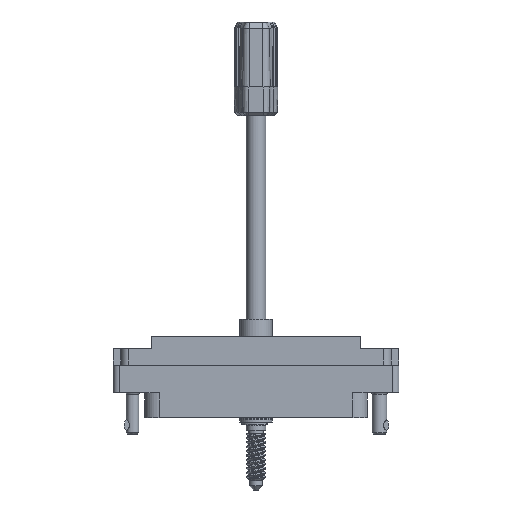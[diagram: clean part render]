
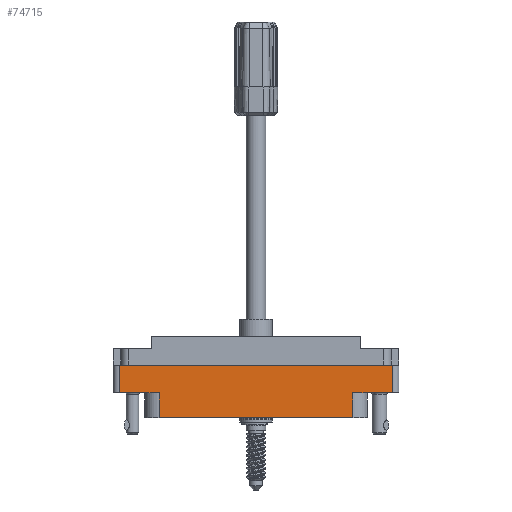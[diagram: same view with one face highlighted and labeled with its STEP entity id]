
A CAD part, front view. The second image highlights one B-rep face of the part: STEP entity #74715.
In plain terms, the highlighted planar face has unit normal (0, -1, 0).
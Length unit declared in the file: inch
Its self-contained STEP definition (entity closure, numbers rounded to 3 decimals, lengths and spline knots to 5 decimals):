
#3395 = EDGE_CURVE ( 'NONE', #43160, #16529, #80920, .T. ) ;
#5774 = DIRECTION ( 'NONE',  ( 0., 0., -1. ) ) ;
#6785 = VECTOR ( 'NONE', #91387, 39.37008 ) ;
#10369 = CARTESIAN_POINT ( 'NONE',  ( 0.9315, -0.7625, -0.54 ) ) ;
#13377 = ORIENTED_EDGE ( 'NONE', *, *, #15025, .T. ) ;
#14695 = CARTESIAN_POINT ( 'NONE',  ( 0., -0.7625, -0.274 ) ) ;
#15025 = EDGE_CURVE ( 'NONE', #37124, #68541, #70095, .T. ) ;
#16529 = VERTEX_POINT ( 'NONE', #10369 ) ;
#18017 = LINE ( 'NONE', #14695, #76082 ) ;
#18328 = EDGE_LOOP ( 'NONE', ( #31202, #13377, #71133, #59614, #92770, #39769, #99316, #72364 ) ) ;
#21700 = DIRECTION ( 'NONE',  ( 0., -1., 0. ) ) ;
#24438 = EDGE_CURVE ( 'NONE', #56185, #54144, #89259, .T. ) ;
#24839 = CARTESIAN_POINT ( 'NONE',  ( 1.313, -0.7625, -0.54 ) ) ;
#24849 = CARTESIAN_POINT ( 'NONE',  ( -0.9315, -0.7625, -0.54 ) ) ;
#25335 = EDGE_CURVE ( 'NONE', #37124, #78351, #18017, .T. ) ;
#25535 = AXIS2_PLACEMENT_3D ( 'NONE', #71431, #21700, #5774 ) ;
#26739 = DIRECTION ( 'NONE',  ( 1., 0., 0. ) ) ;
#31202 = ORIENTED_EDGE ( 'NONE', *, *, #25335, .F. ) ;
#31685 = CARTESIAN_POINT ( 'NONE',  ( 1.313, -0.7625, -0.274 ) ) ;
#31794 = EDGE_CURVE ( 'NONE', #68541, #56185, #71143, .T. ) ;
#32706 = CARTESIAN_POINT ( 'NONE',  ( -1.313, -0.7625, -0.54 ) ) ;
#33283 = CARTESIAN_POINT ( 'NONE',  ( 0., -0.7625, -0.54 ) ) ;
#37124 = VERTEX_POINT ( 'NONE', #56682 ) ;
#39769 = ORIENTED_EDGE ( 'NONE', *, *, #3395, .T. ) ;
#41901 = CARTESIAN_POINT ( 'NONE',  ( -0.9315, -0.7625, -0.78 ) ) ;
#43160 = VERTEX_POINT ( 'NONE', #103483 ) ;
#44789 = VECTOR ( 'NONE', #91651, 39.37008 ) ;
#46068 = DIRECTION ( 'NONE',  ( 0., 0., -1. ) ) ;
#46849 = LINE ( 'NONE', #48165, #6785 ) ;
#48165 = CARTESIAN_POINT ( 'NONE',  ( -1.375, -0.7625, -0.78 ) ) ;
#49703 = LINE ( 'NONE', #74828, #88443 ) ;
#54144 = VERTEX_POINT ( 'NONE', #41901 ) ;
#56185 = VERTEX_POINT ( 'NONE', #24849 ) ;
#56682 = CARTESIAN_POINT ( 'NONE',  ( -1.313, -0.7625, -0.274 ) ) ;
#58625 = VERTEX_POINT ( 'NONE', #24839 ) ;
#59614 = ORIENTED_EDGE ( 'NONE', *, *, #24438, .T. ) ;
#60328 = VECTOR ( 'NONE', #91038, 39.37008 ) ;
#62962 = LINE ( 'NONE', #33283, #60328 ) ;
#65207 = DIRECTION ( 'NONE',  ( 0., 0., -1. ) ) ;
#66833 = DIRECTION ( 'NONE',  ( 0., 0., 1. ) ) ;
#67616 = EDGE_CURVE ( 'NONE', #58625, #16529, #62962, .T. ) ;
#68541 = VERTEX_POINT ( 'NONE', #32706 ) ;
#70095 = LINE ( 'NONE', #105272, #94641 ) ;
#71133 = ORIENTED_EDGE ( 'NONE', *, *, #31794, .T. ) ;
#71143 = LINE ( 'NONE', #76127, #78869 ) ;
#71431 = CARTESIAN_POINT ( 'NONE',  ( -1.375, -0.7625, -0.78 ) ) ;
#72364 = ORIENTED_EDGE ( 'NONE', *, *, #103157, .T. ) ;
#72383 = FACE_OUTER_BOUND ( 'NONE', #18328, .T. ) ;
#73969 = CARTESIAN_POINT ( 'NONE',  ( 0.9315, -0.7625, -0.54 ) ) ;
#74715 = ADVANCED_FACE ( 'NONE', ( #72383 ), #105742, .T. ) ;
#74828 = CARTESIAN_POINT ( 'NONE',  ( 1.313, -0.7625, -0.78 ) ) ;
#76082 = VECTOR ( 'NONE', #105280, 39.37008 ) ;
#76127 = CARTESIAN_POINT ( 'NONE',  ( 0., -0.7625, -0.54 ) ) ;
#78351 = VERTEX_POINT ( 'NONE', #31685 ) ;
#78869 = VECTOR ( 'NONE', #26739, 39.37008 ) ;
#80920 = LINE ( 'NONE', #73969, #44789 ) ;
#85428 = VECTOR ( 'NONE', #65207, 39.37008 ) ;
#88443 = VECTOR ( 'NONE', #66833, 39.37008 ) ;
#89259 = LINE ( 'NONE', #106081, #85428 ) ;
#91038 = DIRECTION ( 'NONE',  ( -1., 0., 0. ) ) ;
#91387 = DIRECTION ( 'NONE',  ( 1., 0., 0. ) ) ;
#91651 = DIRECTION ( 'NONE',  ( 0., 0., 1. ) ) ;
#92770 = ORIENTED_EDGE ( 'NONE', *, *, #99794, .T. ) ;
#94641 = VECTOR ( 'NONE', #46068, 39.37008 ) ;
#99316 = ORIENTED_EDGE ( 'NONE', *, *, #67616, .F. ) ;
#99794 = EDGE_CURVE ( 'NONE', #54144, #43160, #46849, .T. ) ;
#103157 = EDGE_CURVE ( 'NONE', #58625, #78351, #49703, .T. ) ;
#103483 = CARTESIAN_POINT ( 'NONE',  ( 0.9315, -0.7625, -0.78 ) ) ;
#105272 = CARTESIAN_POINT ( 'NONE',  ( -1.313, -0.7625, -0.78 ) ) ;
#105280 = DIRECTION ( 'NONE',  ( 1., 0., 0. ) ) ;
#105742 = PLANE ( 'NONE',  #25535 ) ;
#106081 = CARTESIAN_POINT ( 'NONE',  ( -0.9315, -0.7625, -0.78 ) ) ;
